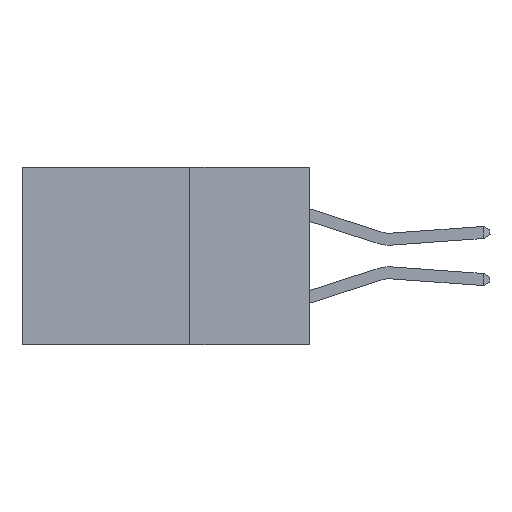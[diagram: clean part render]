
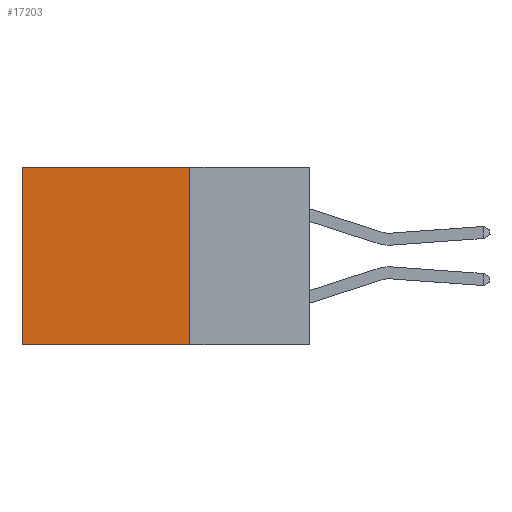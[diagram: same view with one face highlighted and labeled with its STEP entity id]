
A CAD part, left-side view. The second image highlights one B-rep face of the part: STEP entity #17203.
In plain terms, the highlighted planar face has unit normal (-1, 0, 0).
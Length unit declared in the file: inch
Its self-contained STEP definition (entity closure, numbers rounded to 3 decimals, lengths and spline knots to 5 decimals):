
#342 = EDGE_CURVE ( 'NONE', #9731, #24640, #18534, .T. ) ;
#356 = CARTESIAN_POINT ( 'NONE',  ( 0.2615, 0.25, -0.37 ) ) ;
#1773 = DIRECTION ( 'NONE',  ( 0., 0., -1. ) ) ;
#2483 = DIRECTION ( 'NONE',  ( 0., 0., -1. ) ) ;
#2838 = VECTOR ( 'NONE', #1773, 39.37008 ) ;
#2939 = EDGE_CURVE ( 'NONE', #4521, #9731, #6474, .T. ) ;
#4439 = ORIENTED_EDGE ( 'NONE', *, *, #16897, .T. ) ;
#4521 = VERTEX_POINT ( 'NONE', #9587 ) ;
#4611 = VECTOR ( 'NONE', #24575, 39.37008 ) ;
#5931 = VECTOR ( 'NONE', #15859, 39.37008 ) ;
#6167 = LINE ( 'NONE', #25869, #5931 ) ;
#6474 = LINE ( 'NONE', #12442, #21329 ) ;
#8801 = CARTESIAN_POINT ( 'NONE',  ( 0.2615, 0.6, -0.37 ) ) ;
#8852 = CARTESIAN_POINT ( 'NONE',  ( 0.2615, 0.25, -0.37 ) ) ;
#9131 = EDGE_CURVE ( 'NONE', #13858, #24640, #9738, .T. ) ;
#9587 = CARTESIAN_POINT ( 'NONE',  ( 0.2615, 0.25, 0. ) ) ;
#9731 = VERTEX_POINT ( 'NONE', #12853 ) ;
#9738 = LINE ( 'NONE', #25837, #2838 ) ;
#11455 = ORIENTED_EDGE ( 'NONE', *, *, #2939, .F. ) ;
#12439 = PLANE ( 'NONE',  #16549 ) ;
#12442 = CARTESIAN_POINT ( 'NONE',  ( 0.2615, 0.25, -0.37 ) ) ;
#12853 = CARTESIAN_POINT ( 'NONE',  ( 0.2615, 0.25, -0.37 ) ) ;
#13858 = VERTEX_POINT ( 'NONE', #25451 ) ;
#14560 = FACE_OUTER_BOUND ( 'NONE', #15280, .T. ) ;
#15280 = EDGE_LOOP ( 'NONE', ( #18415, #22404, #11455, #4439 ) ) ;
#15859 = DIRECTION ( 'NONE',  ( 0., 1., 0. ) ) ;
#16549 = AXIS2_PLACEMENT_3D ( 'NONE', #8852, #22881, #20379 ) ;
#16897 = EDGE_CURVE ( 'NONE', #4521, #13858, #6167, .T. ) ;
#17203 = ADVANCED_FACE ( 'NONE', ( #14560 ), #12439, .F. ) ;
#18415 = ORIENTED_EDGE ( 'NONE', *, *, #9131, .T. ) ;
#18534 = LINE ( 'NONE', #356, #4611 ) ;
#20379 = DIRECTION ( 'NONE',  ( 0., 0., -1. ) ) ;
#21329 = VECTOR ( 'NONE', #2483, 39.37008 ) ;
#22404 = ORIENTED_EDGE ( 'NONE', *, *, #342, .F. ) ;
#22881 = DIRECTION ( 'NONE',  ( 1., 0., 0. ) ) ;
#24575 = DIRECTION ( 'NONE',  ( 0., 1., 0. ) ) ;
#24640 = VERTEX_POINT ( 'NONE', #8801 ) ;
#25451 = CARTESIAN_POINT ( 'NONE',  ( 0.2615, 0.6, 0. ) ) ;
#25837 = CARTESIAN_POINT ( 'NONE',  ( 0.2615, 0.6, -0.37 ) ) ;
#25869 = CARTESIAN_POINT ( 'NONE',  ( 0.2615, 0.25, 0. ) ) ;
